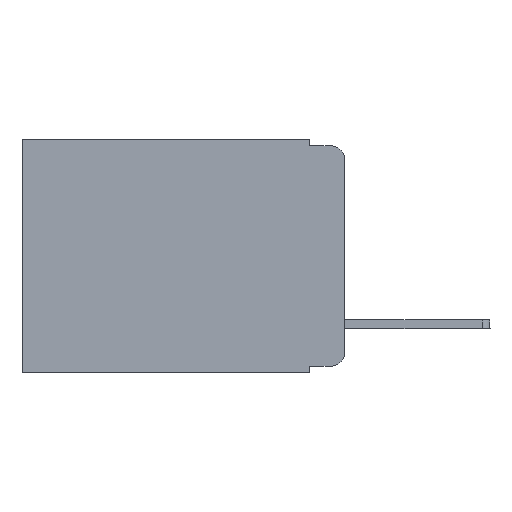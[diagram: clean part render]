
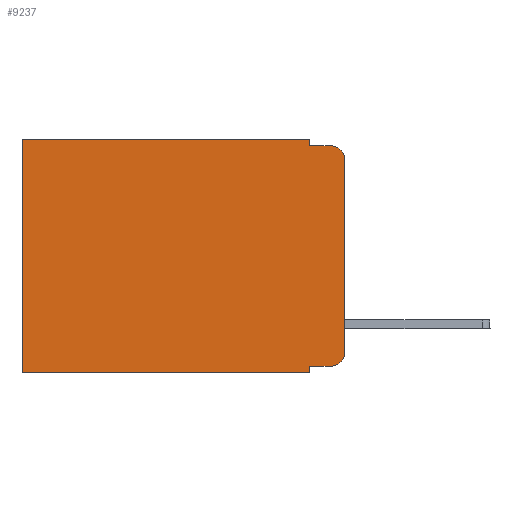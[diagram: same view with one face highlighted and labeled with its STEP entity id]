
A CAD part, left-side view. The second image highlights one B-rep face of the part: STEP entity #9237.
In plain terms, the highlighted planar face has unit normal (-1, 0, 0).
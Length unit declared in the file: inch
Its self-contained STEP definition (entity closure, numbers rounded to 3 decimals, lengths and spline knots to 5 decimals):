
#9 = ORIENTED_EDGE ( 'NONE', *, *, #18524, .F. ) ;
#71 = LINE ( 'NONE', #825, #3128 ) ;
#207 = ORIENTED_EDGE ( 'NONE', *, *, #2084, .F. ) ;
#689 = ORIENTED_EDGE ( 'NONE', *, *, #15790, .F. ) ;
#824 = VECTOR ( 'NONE', #9643, 39.37008 ) ;
#825 = CARTESIAN_POINT ( 'NONE',  ( 0.298, 0.473, 0. ) ) ;
#1272 = VERTEX_POINT ( 'NONE', #15544 ) ;
#1372 = DIRECTION ( 'NONE',  ( 0., 0., -1. ) ) ;
#1378 = EDGE_CURVE ( 'NONE', #18416, #17599, #9535, .T. ) ;
#1596 = ORIENTED_EDGE ( 'NONE', *, *, #12325, .T. ) ;
#1634 = CARTESIAN_POINT ( 'NONE',  ( 0.298, 0., 0. ) ) ;
#2084 = EDGE_CURVE ( 'NONE', #16196, #17599, #9978, .T. ) ;
#2162 = CARTESIAN_POINT ( 'NONE',  ( 0.298, 0., -0.03 ) ) ;
#2200 = LINE ( 'NONE', #6062, #7598 ) ;
#2606 = EDGE_LOOP ( 'NONE', ( #207, #10238, #14176, #689, #1596, #2613, #17972, #9, #11506, #9853 ) ) ;
#2613 = ORIENTED_EDGE ( 'NONE', *, *, #17941, .T. ) ;
#2704 = DIRECTION ( 'NONE',  ( 0., -1., 0. ) ) ;
#2856 = CARTESIAN_POINT ( 'NONE',  ( 0.298, 0.473, 0. ) ) ;
#3128 = VECTOR ( 'NONE', #12884, 39.37008 ) ;
#3158 = CARTESIAN_POINT ( 'NONE',  ( 0.298, 0.051, 0. ) ) ;
#3908 = LINE ( 'NONE', #5427, #16642 ) ;
#4076 = LINE ( 'NONE', #3158, #9730 ) ;
#4535 = LINE ( 'NONE', #5680, #9696 ) ;
#5369 = VERTEX_POINT ( 'NONE', #12233 ) ;
#5427 = CARTESIAN_POINT ( 'NONE',  ( 0.298, 0.051, -0.333 ) ) ;
#5680 = CARTESIAN_POINT ( 'NONE',  ( 0.298, 0.051, 0. ) ) ;
#5983 = LINE ( 'NONE', #13285, #12174 ) ;
#6062 = CARTESIAN_POINT ( 'NONE',  ( 0.298, 0.051, -0.01 ) ) ;
#6217 = CARTESIAN_POINT ( 'NONE',  ( 0.298, 0., -0.313 ) ) ;
#6315 = CARTESIAN_POINT ( 'NONE',  ( 0.298, 0., 0. ) ) ;
#6693 = DIRECTION ( 'NONE',  ( 0., 0., -1. ) ) ;
#6767 = DIRECTION ( 'NONE',  ( -1., 0., 0. ) ) ;
#7452 = CARTESIAN_POINT ( 'NONE',  ( 0.298, 0.051, 0. ) ) ;
#7470 = LINE ( 'NONE', #19320, #11048 ) ;
#7598 = VECTOR ( 'NONE', #7743, 39.37008 ) ;
#7743 = DIRECTION ( 'NONE',  ( 0., -1., 0. ) ) ;
#8301 = CARTESIAN_POINT ( 'NONE',  ( 0.298, 0.02, -0.313 ) ) ;
#8619 = EDGE_CURVE ( 'NONE', #12790, #18416, #3908, .T. ) ;
#9172 = DIRECTION ( 'NONE',  ( 0., 0., -1. ) ) ;
#9237 = ADVANCED_FACE ( 'NONE', ( #9520 ), #13890, .F. ) ;
#9520 = FACE_OUTER_BOUND ( 'NONE', #2606, .T. ) ;
#9535 = CIRCLE ( 'NONE', #13449, 0.02 ) ;
#9643 = DIRECTION ( 'NONE',  ( 0., 0., -1. ) ) ;
#9696 = VECTOR ( 'NONE', #1372, 39.37008 ) ;
#9713 = DIRECTION ( 'NONE',  ( -1., 0., 0. ) ) ;
#9730 = VECTOR ( 'NONE', #18314, 39.37008 ) ;
#9853 = ORIENTED_EDGE ( 'NONE', *, *, #1378, .T. ) ;
#9901 = CARTESIAN_POINT ( 'NONE',  ( 0.298, 0.02, -0.03 ) ) ;
#9978 = LINE ( 'NONE', #1634, #824 ) ;
#10154 = DIRECTION ( 'NONE',  ( 0., 1., 0. ) ) ;
#10238 = ORIENTED_EDGE ( 'NONE', *, *, #13227, .T. ) ;
#10811 = EDGE_CURVE ( 'NONE', #15444, #18921, #7470, .T. ) ;
#11026 = CARTESIAN_POINT ( 'NONE',  ( 0.298, 0.051, -0.343 ) ) ;
#11048 = VECTOR ( 'NONE', #10154, 39.37008 ) ;
#11412 = CARTESIAN_POINT ( 'NONE',  ( 0.298, 0.051, -0.333 ) ) ;
#11506 = ORIENTED_EDGE ( 'NONE', *, *, #8619, .T. ) ;
#11935 = CARTESIAN_POINT ( 'NONE',  ( 0.298, 0.02, -0.333 ) ) ;
#11966 = DIRECTION ( 'NONE',  ( 0., 1., 0. ) ) ;
#12174 = VECTOR ( 'NONE', #11966, 39.37008 ) ;
#12233 = CARTESIAN_POINT ( 'NONE',  ( 0.298, 0.02, -0.01 ) ) ;
#12325 = EDGE_CURVE ( 'NONE', #13898, #12328, #5983, .T. ) ;
#12328 = VERTEX_POINT ( 'NONE', #2856 ) ;
#12790 = VERTEX_POINT ( 'NONE', #11412 ) ;
#12884 = DIRECTION ( 'NONE',  ( 0., 0., -1. ) ) ;
#13227 = EDGE_CURVE ( 'NONE', #16196, #5369, #14302, .T. ) ;
#13285 = CARTESIAN_POINT ( 'NONE',  ( 0.298, 0., 0. ) ) ;
#13449 = AXIS2_PLACEMENT_3D ( 'NONE', #8301, #6767, #6693 ) ;
#13890 = PLANE ( 'NONE',  #18767 ) ;
#13898 = VERTEX_POINT ( 'NONE', #7452 ) ;
#14176 = ORIENTED_EDGE ( 'NONE', *, *, #17891, .F. ) ;
#14294 = DIRECTION ( 'NONE',  ( 0., 0., -1. ) ) ;
#14302 = CIRCLE ( 'NONE', #19541, 0.02 ) ;
#15444 = VERTEX_POINT ( 'NONE', #11026 ) ;
#15544 = CARTESIAN_POINT ( 'NONE',  ( 0.298, 0.051, -0.01 ) ) ;
#15790 = EDGE_CURVE ( 'NONE', #13898, #1272, #4535, .T. ) ;
#16196 = VERTEX_POINT ( 'NONE', #2162 ) ;
#16642 = VECTOR ( 'NONE', #2704, 39.37008 ) ;
#16785 = DIRECTION ( 'NONE',  ( 1., 0., 0. ) ) ;
#17599 = VERTEX_POINT ( 'NONE', #6217 ) ;
#17833 = CARTESIAN_POINT ( 'NONE',  ( 0.298, 0.473, -0.343 ) ) ;
#17891 = EDGE_CURVE ( 'NONE', #1272, #5369, #2200, .T. ) ;
#17941 = EDGE_CURVE ( 'NONE', #12328, #18921, #71, .T. ) ;
#17972 = ORIENTED_EDGE ( 'NONE', *, *, #10811, .F. ) ;
#18314 = DIRECTION ( 'NONE',  ( 0., 0., -1. ) ) ;
#18416 = VERTEX_POINT ( 'NONE', #11935 ) ;
#18524 = EDGE_CURVE ( 'NONE', #12790, #15444, #4076, .T. ) ;
#18767 = AXIS2_PLACEMENT_3D ( 'NONE', #6315, #16785, #9172 ) ;
#18921 = VERTEX_POINT ( 'NONE', #17833 ) ;
#19320 = CARTESIAN_POINT ( 'NONE',  ( 0.298, 0., -0.343 ) ) ;
#19541 = AXIS2_PLACEMENT_3D ( 'NONE', #9901, #9713, #14294 ) ;
